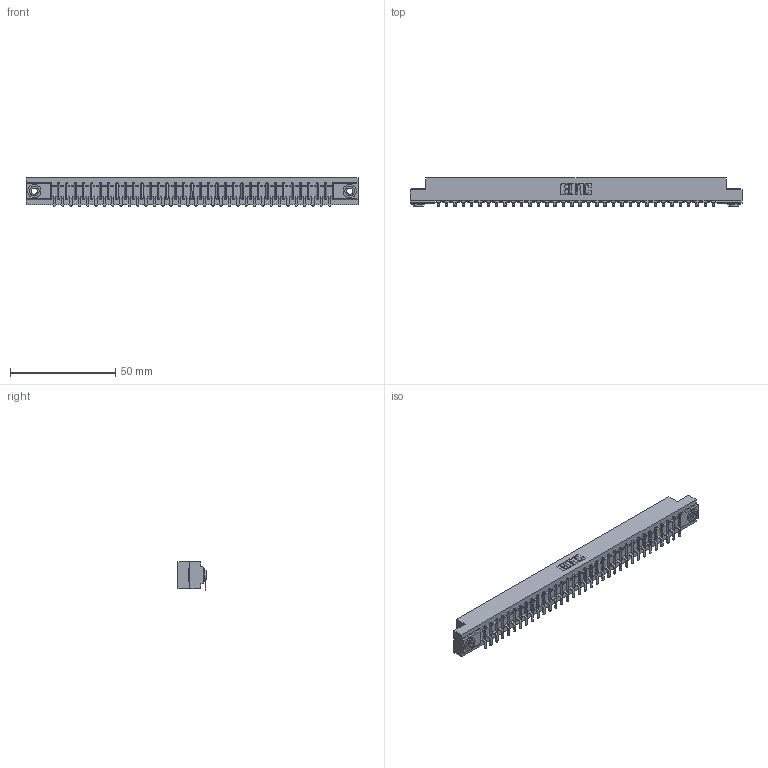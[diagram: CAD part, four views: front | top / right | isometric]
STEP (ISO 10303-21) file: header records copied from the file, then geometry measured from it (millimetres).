
FILE_DESCRIPTION (( 'STEP AP203' ), '1' );
FILE_NAME ('307-034-553-103.STEP', '2018-08-05T01:14:18', ( '' ), ( '' ), 'SwSTEP 2.0', 'SolidWorks 2016', '' );
FILE_SCHEMA (( 'CONFIG_CONTROL_DESIGN' ));
Length unit declared in the file: inch
Products named in the file (4): 307-290-002_553; 345-250-002_345-250-002-102; 307-034-553-103; 307 Part_.156 Dia Mounting Holes
Assembly tree (37 placements, depth 2):
  307-034-553-103
    307 Part_.156 Dia Mounting Holes
    307-290-002_553  x34
    345-250-002_345-250-002-102  x2
Bounding box: 157.73 x 13.36 x 13.5 mm (x, y, z)
Volume: 16821 mm3; surface area: 21218.5 mm2
Topology: 37 solids, 37 shells, 2857 faces, 8731 edges, 5722 vertices
Faces by surface type: plane 1692, cylinder 1087, sphere 70, cone 8
Entity records: 32053 total; most frequent: CARTESIAN_POINT 5385, ORIENTED_EDGE 5366, DIRECTION 5251, EDGE_CURVE 2683, VECTOR 2043, LINE 2043, VERTEX_POINT 1738, AXIS2_PLACEMENT_3D 1604
